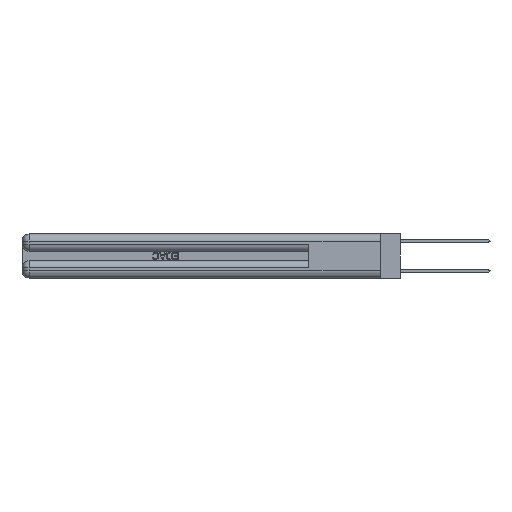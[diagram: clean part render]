
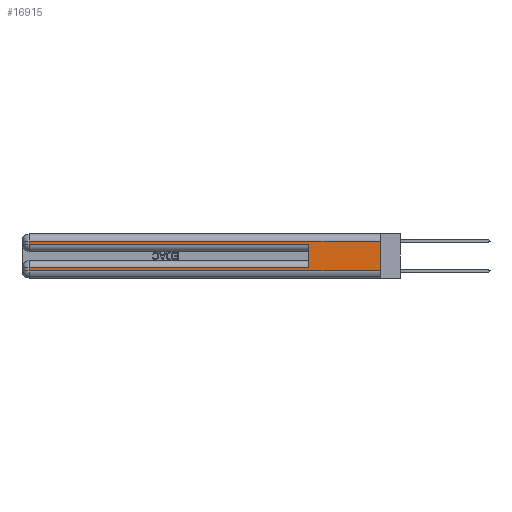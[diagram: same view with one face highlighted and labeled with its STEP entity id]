
A CAD part, left-side view. The second image highlights one B-rep face of the part: STEP entity #16915.
In plain terms, the highlighted planar face has unit normal (-1, 0, 0).
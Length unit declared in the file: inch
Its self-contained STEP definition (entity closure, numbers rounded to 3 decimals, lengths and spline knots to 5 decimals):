
#302 = LINE ( 'NONE', #31998, #20916 ) ;
#362 = CARTESIAN_POINT ( 'NONE',  ( 0., 2.94, 0.285 ) ) ;
#468 = ORIENTED_EDGE ( 'NONE', *, *, #22717, .T. ) ;
#520 = LINE ( 'NONE', #21127, #14021 ) ;
#1445 = VERTEX_POINT ( 'NONE', #7567 ) ;
#2743 = ORIENTED_EDGE ( 'NONE', *, *, #24526, .T. ) ;
#3459 = AXIS2_PLACEMENT_3D ( 'NONE', #3779, #11979, #30786 ) ;
#3779 = CARTESIAN_POINT ( 'NONE',  ( 0., 0., 0.37 ) ) ;
#3810 = LINE ( 'NONE', #24088, #23509 ) ;
#4633 = LINE ( 'NONE', #5862, #18076 ) ;
#4741 = EDGE_CURVE ( 'NONE', #1445, #33214, #3810, .T. ) ;
#5862 = CARTESIAN_POINT ( 'NONE',  ( 0., 0., 0.31 ) ) ;
#7567 = CARTESIAN_POINT ( 'NONE',  ( 0., 0.6, 0.085 ) ) ;
#8104 = CARTESIAN_POINT ( 'NONE',  ( 0., 0., 0.31 ) ) ;
#8570 = DIRECTION ( 'NONE',  ( 0., 1., 0. ) ) ;
#8599 = VERTEX_POINT ( 'NONE', #31702 ) ;
#8827 = DIRECTION ( 'NONE',  ( 0., -1., 0. ) ) ;
#10092 = CARTESIAN_POINT ( 'NONE',  ( 0., 2.94, 0.31 ) ) ;
#10138 = EDGE_CURVE ( 'NONE', #20261, #33550, #302, .T. ) ;
#10398 = VECTOR ( 'NONE', #33103, 39.37008 ) ;
#11979 = DIRECTION ( 'NONE',  ( 1., 0., 0. ) ) ;
#12805 = LINE ( 'NONE', #19590, #19093 ) ;
#13655 = VERTEX_POINT ( 'NONE', #29774 ) ;
#14021 = VECTOR ( 'NONE', #26543, 39.37008 ) ;
#14378 = ORIENTED_EDGE ( 'NONE', *, *, #16247, .T. ) ;
#15278 = VECTOR ( 'NONE', #19109, 39.37008 ) ;
#15952 = VECTOR ( 'NONE', #8827, 39.37008 ) ;
#16131 = LINE ( 'NONE', #16441, #15278 ) ;
#16160 = DIRECTION ( 'NONE',  ( 0., 0., 1. ) ) ;
#16247 = EDGE_CURVE ( 'NONE', #13655, #33550, #17591, .T. ) ;
#16441 = CARTESIAN_POINT ( 'NONE',  ( 0., 0., 0.285 ) ) ;
#16915 = ADVANCED_FACE ( 'NONE', ( #29716 ), #22633, .F. ) ;
#17022 = CARTESIAN_POINT ( 'NONE',  ( 0., 0., 0.085 ) ) ;
#17591 = LINE ( 'NONE', #19409, #15952 ) ;
#18076 = VECTOR ( 'NONE', #8570, 39.37008 ) ;
#19093 = VECTOR ( 'NONE', #30417, 39.37008 ) ;
#19109 = DIRECTION ( 'NONE',  ( 0., -1., 0. ) ) ;
#19409 = CARTESIAN_POINT ( 'NONE',  ( 0., 0., 0.06 ) ) ;
#19590 = CARTESIAN_POINT ( 'NONE',  ( 0., 2.94, 0.37 ) ) ;
#19661 = CARTESIAN_POINT ( 'NONE',  ( 0., 0.6, 0.285 ) ) ;
#20261 = VERTEX_POINT ( 'NONE', #8104 ) ;
#20916 = VECTOR ( 'NONE', #34701, 39.37008 ) ;
#21127 = CARTESIAN_POINT ( 'NONE',  ( 0., 2.94, 0.37 ) ) ;
#21161 = CARTESIAN_POINT ( 'NONE',  ( 0., 0., 0.06 ) ) ;
#22203 = ORIENTED_EDGE ( 'NONE', *, *, #28809, .T. ) ;
#22633 = PLANE ( 'NONE',  #3459 ) ;
#22717 = EDGE_CURVE ( 'NONE', #34070, #23821, #520, .T. ) ;
#23509 = VECTOR ( 'NONE', #16160, 39.37008 ) ;
#23740 = ORIENTED_EDGE ( 'NONE', *, *, #30626, .T. ) ;
#23821 = VERTEX_POINT ( 'NONE', #362 ) ;
#24088 = CARTESIAN_POINT ( 'NONE',  ( 0., 0.6, 0.145 ) ) ;
#24526 = EDGE_CURVE ( 'NONE', #20261, #34070, #4633, .T. ) ;
#26543 = DIRECTION ( 'NONE',  ( 0., 0., -1. ) ) ;
#27018 = EDGE_CURVE ( 'NONE', #1445, #8599, #31005, .T. ) ;
#28809 = EDGE_CURVE ( 'NONE', #8599, #13655, #12805, .T. ) ;
#29695 = EDGE_LOOP ( 'NONE', ( #31088, #2743, #468, #23740, #29743, #32644, #22203, #14378 ) ) ;
#29716 = FACE_OUTER_BOUND ( 'NONE', #29695, .T. ) ;
#29743 = ORIENTED_EDGE ( 'NONE', *, *, #4741, .F. ) ;
#29774 = CARTESIAN_POINT ( 'NONE',  ( 0., 2.94, 0.06 ) ) ;
#30417 = DIRECTION ( 'NONE',  ( 0., 0., -1. ) ) ;
#30626 = EDGE_CURVE ( 'NONE', #23821, #33214, #16131, .T. ) ;
#30786 = DIRECTION ( 'NONE',  ( 0., 0., -1. ) ) ;
#31005 = LINE ( 'NONE', #17022, #10398 ) ;
#31088 = ORIENTED_EDGE ( 'NONE', *, *, #10138, .F. ) ;
#31702 = CARTESIAN_POINT ( 'NONE',  ( 0., 2.94, 0.085 ) ) ;
#31998 = CARTESIAN_POINT ( 'NONE',  ( 0., 0., 0.37 ) ) ;
#32644 = ORIENTED_EDGE ( 'NONE', *, *, #27018, .T. ) ;
#33103 = DIRECTION ( 'NONE',  ( 0., 1., 0. ) ) ;
#33214 = VERTEX_POINT ( 'NONE', #19661 ) ;
#33550 = VERTEX_POINT ( 'NONE', #21161 ) ;
#34070 = VERTEX_POINT ( 'NONE', #10092 ) ;
#34701 = DIRECTION ( 'NONE',  ( 0., 0., -1. ) ) ;
